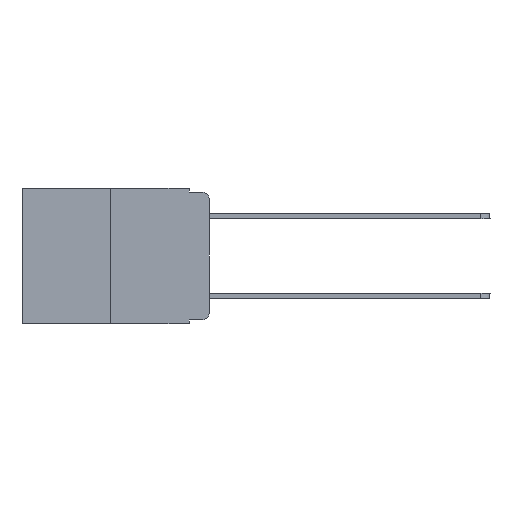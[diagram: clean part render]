
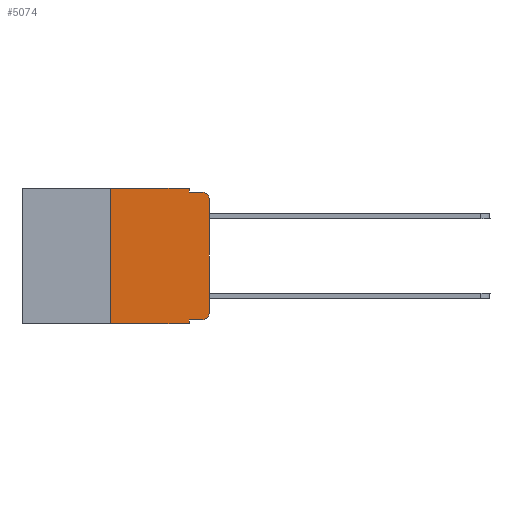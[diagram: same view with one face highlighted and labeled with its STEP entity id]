
A CAD part, left-side view. The second image highlights one B-rep face of the part: STEP entity #5074.
In plain terms, the highlighted planar face has unit normal (-1, 0, 0).
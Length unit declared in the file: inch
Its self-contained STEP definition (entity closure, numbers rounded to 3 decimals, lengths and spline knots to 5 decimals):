
#341 = CARTESIAN_POINT ( 'NONE',  ( 0., 0.051, -0.343 ) ) ;
#373 = VERTEX_POINT ( 'NONE', #4461 ) ;
#557 = VERTEX_POINT ( 'NONE', #16299 ) ;
#867 = ORIENTED_EDGE ( 'NONE', *, *, #5987, .F. ) ;
#1282 = ORIENTED_EDGE ( 'NONE', *, *, #10898, .T. ) ;
#1797 = CARTESIAN_POINT ( 'NONE',  ( 0., 0.02, -0.03 ) ) ;
#2098 = CIRCLE ( 'NONE', #14918, 0.02 ) ;
#2145 = ORIENTED_EDGE ( 'NONE', *, *, #9643, .T. ) ;
#2188 = CARTESIAN_POINT ( 'NONE',  ( 0., 0., -0.03 ) ) ;
#3309 = ORIENTED_EDGE ( 'NONE', *, *, #10588, .F. ) ;
#3393 = ORIENTED_EDGE ( 'NONE', *, *, #8314, .F. ) ;
#3398 = LINE ( 'NONE', #6357, #4224 ) ;
#3455 = CARTESIAN_POINT ( 'NONE',  ( 0., 0.02, -0.333 ) ) ;
#3633 = VERTEX_POINT ( 'NONE', #16549 ) ;
#3781 = EDGE_CURVE ( 'NONE', #11686, #3633, #8533, .T. ) ;
#3807 = DIRECTION ( 'NONE',  ( 0., 0., -1. ) ) ;
#3880 = AXIS2_PLACEMENT_3D ( 'NONE', #10969, #6934, #7102 ) ;
#3956 = VERTEX_POINT ( 'NONE', #7883 ) ;
#4052 = EDGE_CURVE ( 'NONE', #6886, #3956, #2098, .T. ) ;
#4135 = EDGE_CURVE ( 'NONE', #557, #15588, #13573, .T. ) ;
#4224 = VECTOR ( 'NONE', #15470, 39.37008 ) ;
#4318 = FACE_OUTER_BOUND ( 'NONE', #5291, .T. ) ;
#4461 = CARTESIAN_POINT ( 'NONE',  ( 0., 0.051, -0.333 ) ) ;
#5074 = ADVANCED_FACE ( 'NONE', ( #4318 ), #8792, .F. ) ;
#5271 = VECTOR ( 'NONE', #11825, 39.37008 ) ;
#5291 = EDGE_LOOP ( 'NONE', ( #2145, #15976, #867, #6778, #3309, #15732, #5872, #3393, #1282, #14320 ) ) ;
#5305 = CARTESIAN_POINT ( 'NONE',  ( 0., 0.051, 0. ) ) ;
#5382 = CARTESIAN_POINT ( 'NONE',  ( 0., 0.051, -0.01 ) ) ;
#5521 = VECTOR ( 'NONE', #14638, 39.37008 ) ;
#5872 = ORIENTED_EDGE ( 'NONE', *, *, #4135, .T. ) ;
#5987 = EDGE_CURVE ( 'NONE', #3633, #3956, #8455, .T. ) ;
#6357 = CARTESIAN_POINT ( 'NONE',  ( 0., 0.051, -0.333 ) ) ;
#6778 = ORIENTED_EDGE ( 'NONE', *, *, #3781, .F. ) ;
#6825 = CARTESIAN_POINT ( 'NONE',  ( 0., 0.051, 0. ) ) ;
#6886 = VERTEX_POINT ( 'NONE', #2188 ) ;
#6934 = DIRECTION ( 'NONE',  ( -1., 0., 0. ) ) ;
#6959 = EDGE_CURVE ( 'NONE', #557, #7909, #13476, .T. ) ;
#7075 = CARTESIAN_POINT ( 'NONE',  ( 0., 0.473, -0.343 ) ) ;
#7102 = DIRECTION ( 'NONE',  ( 0., 0., -1. ) ) ;
#7883 = CARTESIAN_POINT ( 'NONE',  ( 0., 0.02, -0.01 ) ) ;
#7909 = VERTEX_POINT ( 'NONE', #10844 ) ;
#8314 = EDGE_CURVE ( 'NONE', #373, #15588, #10988, .T. ) ;
#8455 = LINE ( 'NONE', #5382, #5271 ) ;
#8533 = LINE ( 'NONE', #5305, #14202 ) ;
#8792 = PLANE ( 'NONE',  #11667 ) ;
#9166 = VERTEX_POINT ( 'NONE', #3455 ) ;
#9416 = VECTOR ( 'NONE', #12756, 39.37008 ) ;
#9580 = DIRECTION ( 'NONE',  ( 0., 0., -1. ) ) ;
#9643 = EDGE_CURVE ( 'NONE', #11231, #6886, #15718, .T. ) ;
#10222 = EDGE_CURVE ( 'NONE', #9166, #11231, #12883, .T. ) ;
#10588 = EDGE_CURVE ( 'NONE', #7909, #11686, #10638, .T. ) ;
#10638 = LINE ( 'NONE', #12138, #11251 ) ;
#10827 = CARTESIAN_POINT ( 'NONE',  ( 0., 0.051, 0. ) ) ;
#10844 = CARTESIAN_POINT ( 'NONE',  ( 0., 0.25, 0. ) ) ;
#10898 = EDGE_CURVE ( 'NONE', #373, #9166, #3398, .T. ) ;
#10969 = CARTESIAN_POINT ( 'NONE',  ( 0., 0.02, -0.313 ) ) ;
#10988 = LINE ( 'NONE', #10827, #14837 ) ;
#11231 = VERTEX_POINT ( 'NONE', #13707 ) ;
#11251 = VECTOR ( 'NONE', #16143, 39.37008 ) ;
#11667 = AXIS2_PLACEMENT_3D ( 'NONE', #14161, #16604, #3807 ) ;
#11686 = VERTEX_POINT ( 'NONE', #6825 ) ;
#11825 = DIRECTION ( 'NONE',  ( 0., -1., 0. ) ) ;
#12138 = CARTESIAN_POINT ( 'NONE',  ( 0., 0.473, 0. ) ) ;
#12756 = DIRECTION ( 'NONE',  ( 0., 0., 1. ) ) ;
#12883 = CIRCLE ( 'NONE', #3880, 0.02 ) ;
#13373 = DIRECTION ( 'NONE',  ( 0., 0., -1. ) ) ;
#13476 = LINE ( 'NONE', #15242, #9416 ) ;
#13557 = DIRECTION ( 'NONE',  ( -1., 0., 0. ) ) ;
#13573 = LINE ( 'NONE', #7075, #5521 ) ;
#13707 = CARTESIAN_POINT ( 'NONE',  ( 0., 0., -0.313 ) ) ;
#13715 = VECTOR ( 'NONE', #14809, 39.37008 ) ;
#14145 = DIRECTION ( 'NONE',  ( 0., 0., -1. ) ) ;
#14161 = CARTESIAN_POINT ( 'NONE',  ( 0., 0.473, 0. ) ) ;
#14202 = VECTOR ( 'NONE', #14145, 39.37008 ) ;
#14320 = ORIENTED_EDGE ( 'NONE', *, *, #10222, .T. ) ;
#14638 = DIRECTION ( 'NONE',  ( 0., -1., 0. ) ) ;
#14809 = DIRECTION ( 'NONE',  ( 0., 0., 1. ) ) ;
#14837 = VECTOR ( 'NONE', #9580, 39.37008 ) ;
#14918 = AXIS2_PLACEMENT_3D ( 'NONE', #1797, #13557, #13373 ) ;
#15242 = CARTESIAN_POINT ( 'NONE',  ( 0., 0.25, 0. ) ) ;
#15470 = DIRECTION ( 'NONE',  ( 0., -1., 0. ) ) ;
#15588 = VERTEX_POINT ( 'NONE', #341 ) ;
#15718 = LINE ( 'NONE', #16025, #13715 ) ;
#15732 = ORIENTED_EDGE ( 'NONE', *, *, #6959, .F. ) ;
#15976 = ORIENTED_EDGE ( 'NONE', *, *, #4052, .T. ) ;
#16025 = CARTESIAN_POINT ( 'NONE',  ( 0., 0., 0. ) ) ;
#16143 = DIRECTION ( 'NONE',  ( 0., -1., 0. ) ) ;
#16299 = CARTESIAN_POINT ( 'NONE',  ( 0., 0.25, -0.343 ) ) ;
#16549 = CARTESIAN_POINT ( 'NONE',  ( 0., 0.051, -0.01 ) ) ;
#16604 = DIRECTION ( 'NONE',  ( 1., 0., 0. ) ) ;
